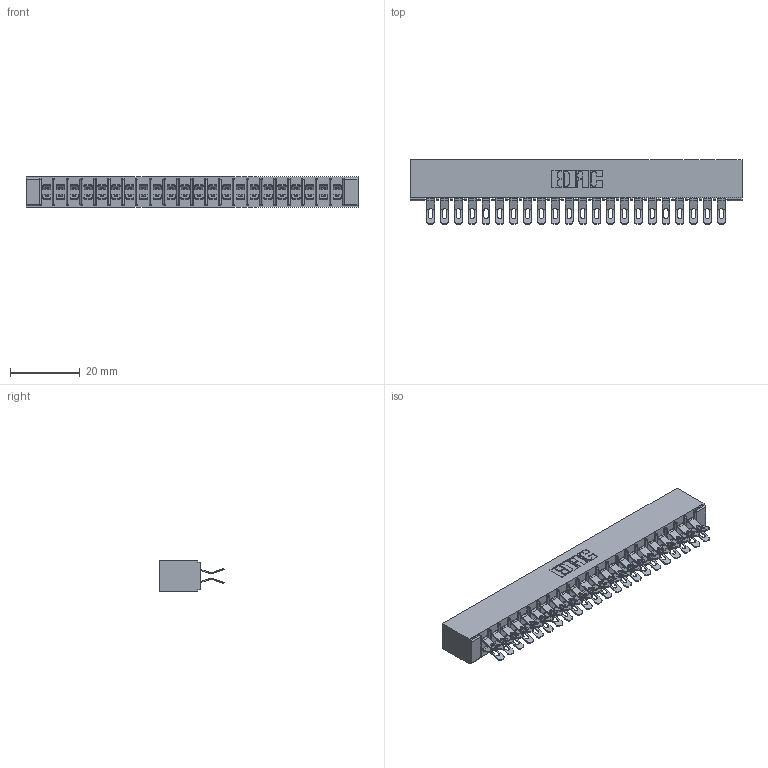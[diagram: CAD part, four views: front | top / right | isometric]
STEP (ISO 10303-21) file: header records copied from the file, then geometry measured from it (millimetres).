
FILE_DESCRIPTION (( 'STEP AP203' ), '1' );
FILE_NAME ('315-044-555-201.STEP', '2019-09-10T17:50:11', ( '' ), ( '' ), 'SwSTEP 2.0', 'SolidWorks 2016', '' );
FILE_SCHEMA (( 'CONFIG_CONTROL_DESIGN' ));
Length unit declared in the file: inch
Products named in the file (3): 315-044-555-201; 305-290-001_555; 305 Part_No Mounting
Assembly tree (45 placements, depth 2):
  315-044-555-201
    305 Part_No Mounting
    305-290-001_555  x44
Bounding box: 95.05 x 18.41 x 8.71 mm (x, y, z)
Volume: 6285.7 mm3; surface area: 13169.4 mm2
Topology: 45 solids, 45 shells, 3012 faces, 8982 edges, 5868 vertices
Faces by surface type: plane 1472, cylinder 1452, sphere 88
Entity records: 26601 total; most frequent: CARTESIAN_POINT 4418, ORIENTED_EDGE 4372, DIRECTION 4282, EDGE_CURVE 2186, VECTOR 1730, LINE 1730, VERTEX_POINT 1396, AXIS2_PLACEMENT_3D 1276
